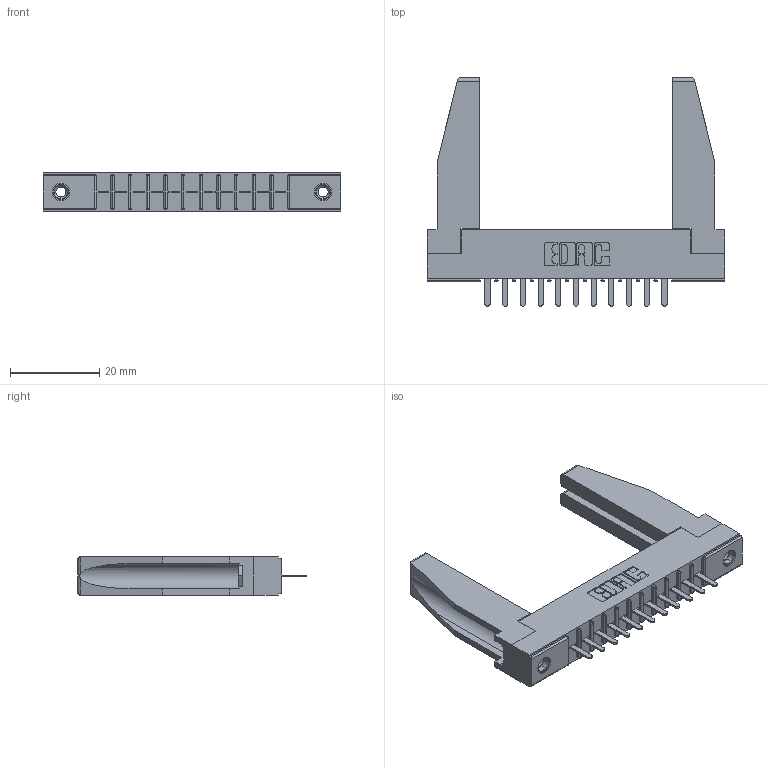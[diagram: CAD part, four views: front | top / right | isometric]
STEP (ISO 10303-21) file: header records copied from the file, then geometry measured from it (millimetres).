
FILE_DESCRIPTION (( 'STEP AP203' ), '1' );
FILE_NAME ('316-011-520-178.STEP', '2018-07-31T00:17:58', ( '' ), ( '' ), 'SwSTEP 2.0', 'SolidWorks 2016', '' );
FILE_SCHEMA (( 'CONFIG_CONTROL_DESIGN' ));
Length unit declared in the file: inch
Products named in the file (5): 316-011-520-178; 306 Part_.156 Dia; 306-290-001_120; 345-250-001_345-250-001-102; 307-220-078
Assembly tree (16 placements, depth 2):
  316-011-520-178
    306 Part_.156 Dia
    306-290-001_120  x11
    345-250-001_345-250-001-102  x2
    307-220-078  x2
Bounding box: 66.6 x 51.16 x 8.71 mm (x, y, z)
Volume: 8505.2 mm3; surface area: 10145.2 mm2
Topology: 16 solids, 16 shells, 1016 faces, 2813 edges, 1806 vertices
Faces by surface type: plane 669, cylinder 287, sphere 44, cone 12, torus 4
Entity records: 16669 total; most frequent: CARTESIAN_POINT 2794, ORIENTED_EDGE 2724, DIRECTION 2710, EDGE_CURVE 1362, VECTOR 1050, LINE 1050, VERTEX_POINT 872, AXIS2_PLACEMENT_3D 830
